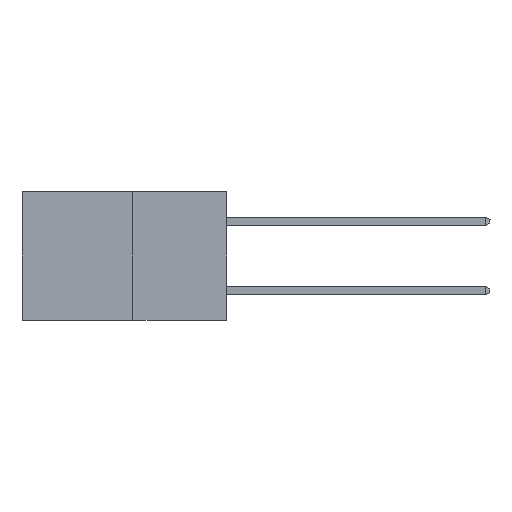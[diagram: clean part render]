
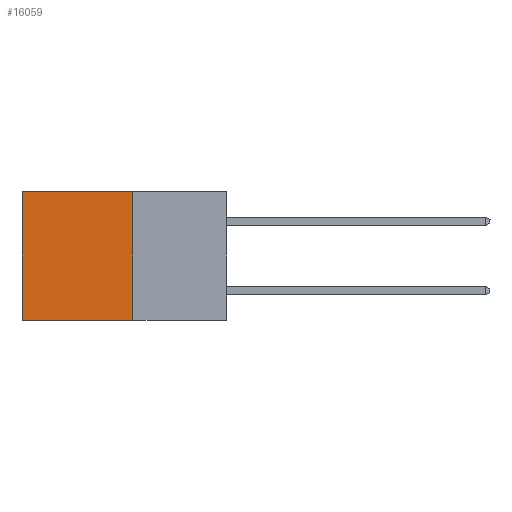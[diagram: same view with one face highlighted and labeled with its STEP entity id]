
A CAD part, left-side view. The second image highlights one B-rep face of the part: STEP entity #16059.
In plain terms, the highlighted planar face has unit normal (-1, 0, 0).
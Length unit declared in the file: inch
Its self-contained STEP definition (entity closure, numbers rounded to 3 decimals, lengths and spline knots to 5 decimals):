
#643 = ORIENTED_EDGE ( 'NONE', *, *, #18096, .T. ) ;
#2854 = EDGE_CURVE ( 'NONE', #12048, #17777, #16757, .T. ) ;
#2972 = VECTOR ( 'NONE', #6688, 39.37008 ) ;
#3000 = ORIENTED_EDGE ( 'NONE', *, *, #16728, .F. ) ;
#4056 = CARTESIAN_POINT ( 'NONE',  ( 0.277, 0.27, 0. ) ) ;
#4759 = CARTESIAN_POINT ( 'NONE',  ( 0.277, 0.27, -0.37 ) ) ;
#5506 = ORIENTED_EDGE ( 'NONE', *, *, #17144, .T. ) ;
#6608 = LINE ( 'NONE', #4056, #14426 ) ;
#6688 = DIRECTION ( 'NONE',  ( 0., 0., -1. ) ) ;
#7142 = LINE ( 'NONE', #19205, #2972 ) ;
#7154 = FACE_OUTER_BOUND ( 'NONE', #19328, .T. ) ;
#7201 = DIRECTION ( 'NONE',  ( 0., 1., 0. ) ) ;
#7404 = PLANE ( 'NONE',  #10506 ) ;
#7943 = VECTOR ( 'NONE', #13919, 39.37008 ) ;
#10365 = VECTOR ( 'NONE', #12123, 39.37008 ) ;
#10506 = AXIS2_PLACEMENT_3D ( 'NONE', #18404, #12079, #19990 ) ;
#10754 = CARTESIAN_POINT ( 'NONE',  ( 0.277, 0.59, 0. ) ) ;
#12048 = VERTEX_POINT ( 'NONE', #4759 ) ;
#12079 = DIRECTION ( 'NONE',  ( 1., 0., 0. ) ) ;
#12123 = DIRECTION ( 'NONE',  ( 0., 0., -1. ) ) ;
#12219 = VERTEX_POINT ( 'NONE', #10754 ) ;
#12252 = CARTESIAN_POINT ( 'NONE',  ( 0.277, 0.27, 0. ) ) ;
#13581 = VERTEX_POINT ( 'NONE', #12252 ) ;
#13919 = DIRECTION ( 'NONE',  ( 0., 1., 0. ) ) ;
#14069 = CARTESIAN_POINT ( 'NONE',  ( 0.277, 0.27, -0.37 ) ) ;
#14426 = VECTOR ( 'NONE', #7201, 39.37008 ) ;
#15690 = ORIENTED_EDGE ( 'NONE', *, *, #2854, .F. ) ;
#16059 = ADVANCED_FACE ( 'NONE', ( #7154 ), #7404, .F. ) ;
#16728 = EDGE_CURVE ( 'NONE', #13581, #12048, #19222, .T. ) ;
#16757 = LINE ( 'NONE', #14069, #7943 ) ;
#17144 = EDGE_CURVE ( 'NONE', #12219, #17777, #7142, .T. ) ;
#17415 = CARTESIAN_POINT ( 'NONE',  ( 0.277, 0.59, -0.37 ) ) ;
#17777 = VERTEX_POINT ( 'NONE', #17415 ) ;
#18096 = EDGE_CURVE ( 'NONE', #13581, #12219, #6608, .T. ) ;
#18377 = CARTESIAN_POINT ( 'NONE',  ( 0.277, 0.27, -0.37 ) ) ;
#18404 = CARTESIAN_POINT ( 'NONE',  ( 0.277, 0.27, -0.37 ) ) ;
#19205 = CARTESIAN_POINT ( 'NONE',  ( 0.277, 0.59, -0.37 ) ) ;
#19222 = LINE ( 'NONE', #18377, #10365 ) ;
#19328 = EDGE_LOOP ( 'NONE', ( #5506, #15690, #3000, #643 ) ) ;
#19990 = DIRECTION ( 'NONE',  ( 0., 0., -1. ) ) ;
